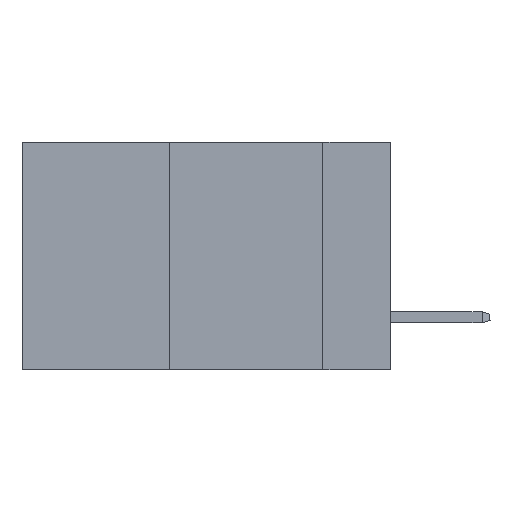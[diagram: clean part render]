
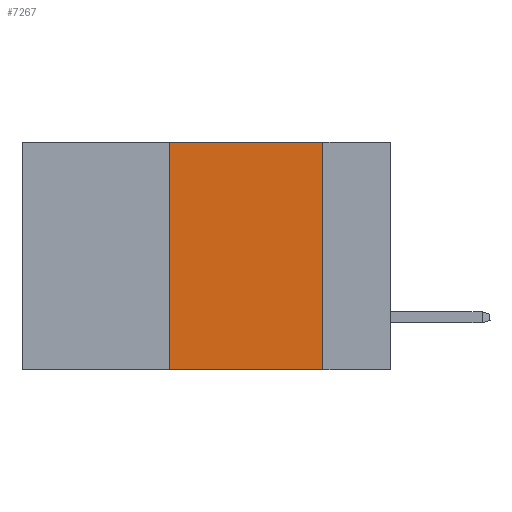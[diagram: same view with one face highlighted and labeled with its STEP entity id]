
A CAD part, left-side view. The second image highlights one B-rep face of the part: STEP entity #7267.
In plain terms, the highlighted planar face has unit normal (-1, 0, 0).
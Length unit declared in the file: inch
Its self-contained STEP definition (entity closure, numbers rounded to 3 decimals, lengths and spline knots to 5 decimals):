
#215 = DIRECTION ( 'NONE',  ( 0., -1., 0. ) ) ;
#627 = DIRECTION ( 'NONE',  ( 0., 0., 1. ) ) ;
#672 = DIRECTION ( 'NONE',  ( 1., 0., 0. ) ) ;
#822 = VERTEX_POINT ( 'NONE', #4786 ) ;
#892 = VECTOR ( 'NONE', #627, 39.37008 ) ;
#1366 = LINE ( 'NONE', #5074, #892 ) ;
#1422 = DIRECTION ( 'NONE',  ( 0., 0., -1. ) ) ;
#1514 = CARTESIAN_POINT ( 'NONE',  ( 0., 0.36, -0.37 ) ) ;
#1636 = ORIENTED_EDGE ( 'NONE', *, *, #5777, .T. ) ;
#2399 = CARTESIAN_POINT ( 'NONE',  ( 0., 0.11, 0. ) ) ;
#2665 = DIRECTION ( 'NONE',  ( 0., 0., -1. ) ) ;
#2879 = CARTESIAN_POINT ( 'NONE',  ( 0., 0.6, 0. ) ) ;
#3232 = VERTEX_POINT ( 'NONE', #2399 ) ;
#3454 = VECTOR ( 'NONE', #2665, 39.37008 ) ;
#3551 = EDGE_CURVE ( 'NONE', #3232, #822, #9569, .T. ) ;
#3827 = EDGE_CURVE ( 'NONE', #8365, #9169, #1366, .T. ) ;
#3867 = DIRECTION ( 'NONE',  ( 0., -1., 0. ) ) ;
#3932 = EDGE_CURVE ( 'NONE', #9169, #3232, #6342, .T. ) ;
#3974 = AXIS2_PLACEMENT_3D ( 'NONE', #2879, #672, #1422 ) ;
#4373 = ORIENTED_EDGE ( 'NONE', *, *, #3827, .F. ) ;
#4786 = CARTESIAN_POINT ( 'NONE',  ( 0., 0.11, -0.37 ) ) ;
#4919 = VECTOR ( 'NONE', #3867, 39.37008 ) ;
#5074 = CARTESIAN_POINT ( 'NONE',  ( 0., 0.36, 0. ) ) ;
#5132 = EDGE_LOOP ( 'NONE', ( #6189, #6934, #4373, #1636 ) ) ;
#5777 = EDGE_CURVE ( 'NONE', #8365, #822, #7231, .T. ) ;
#5859 = PLANE ( 'NONE',  #3974 ) ;
#6189 = ORIENTED_EDGE ( 'NONE', *, *, #3551, .F. ) ;
#6342 = LINE ( 'NONE', #6851, #7488 ) ;
#6851 = CARTESIAN_POINT ( 'NONE',  ( 0., 0.6, 0. ) ) ;
#6934 = ORIENTED_EDGE ( 'NONE', *, *, #3932, .F. ) ;
#7120 = CARTESIAN_POINT ( 'NONE',  ( 0., 0.11, 0. ) ) ;
#7231 = LINE ( 'NONE', #8385, #4919 ) ;
#7267 = ADVANCED_FACE ( 'NONE', ( #9003 ), #5859, .F. ) ;
#7488 = VECTOR ( 'NONE', #215, 39.37008 ) ;
#8019 = CARTESIAN_POINT ( 'NONE',  ( 0., 0.36, 0. ) ) ;
#8365 = VERTEX_POINT ( 'NONE', #1514 ) ;
#8385 = CARTESIAN_POINT ( 'NONE',  ( 0., 0.6, -0.37 ) ) ;
#9003 = FACE_OUTER_BOUND ( 'NONE', #5132, .T. ) ;
#9169 = VERTEX_POINT ( 'NONE', #8019 ) ;
#9569 = LINE ( 'NONE', #7120, #3454 ) ;
